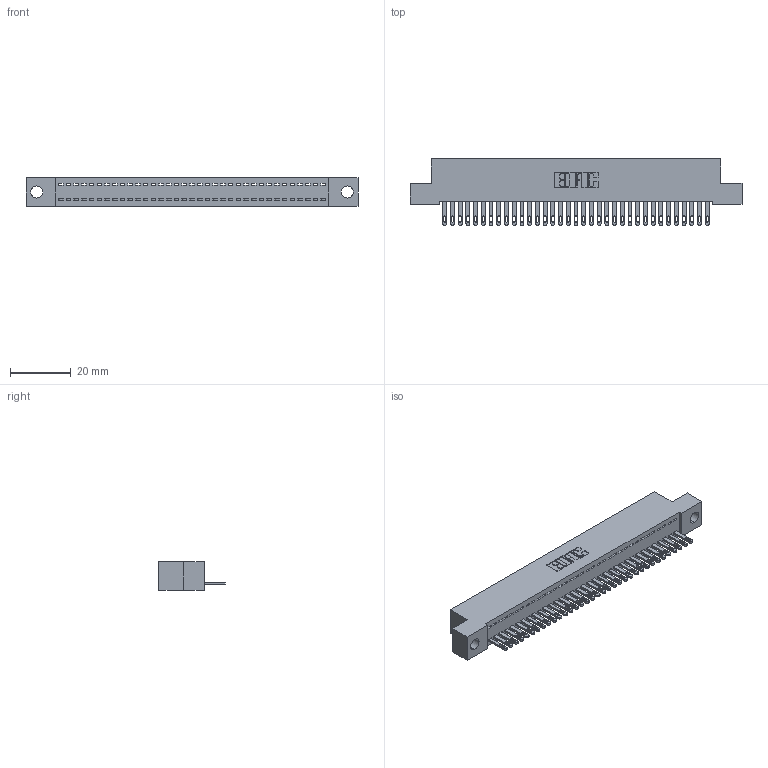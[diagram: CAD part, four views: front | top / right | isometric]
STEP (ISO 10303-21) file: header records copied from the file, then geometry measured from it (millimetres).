
FILE_DESCRIPTION (( 'STEP AP203' ), '1' );
FILE_NAME ('342-035-500-104.STEP', '2019-10-02T12:40:31', ( '' ), ( '' ), 'SwSTEP 2.0', 'SolidWorks 2016', '' );
FILE_SCHEMA (( 'CONFIG_CONTROL_DESIGN' ));
Length unit declared in the file: inch
Products named in the file (3): 342 Part_.156 TH; 345-292-001_345-293-100; 342-035-500-104
Assembly tree (36 placements, depth 2):
  342-035-500-104
    342 Part_.156 TH
    345-292-001_345-293-100  x35
Bounding box: 109.22 x 21.85 x 9.4 mm (x, y, z)
Volume: 9485.3 mm3; surface area: 13685.7 mm2
Topology: 36 solids, 36 shells, 2000 faces, 6179 edges, 4118 vertices
Faces by surface type: plane 1326, cylinder 674
Entity records: 22103 total; most frequent: CARTESIAN_POINT 3819, ORIENTED_EDGE 3790, DIRECTION 3237, EDGE_CURVE 1895, VECTOR 1763, LINE 1763, VERTEX_POINT 1262, AXIS2_PLACEMENT_3D 737
